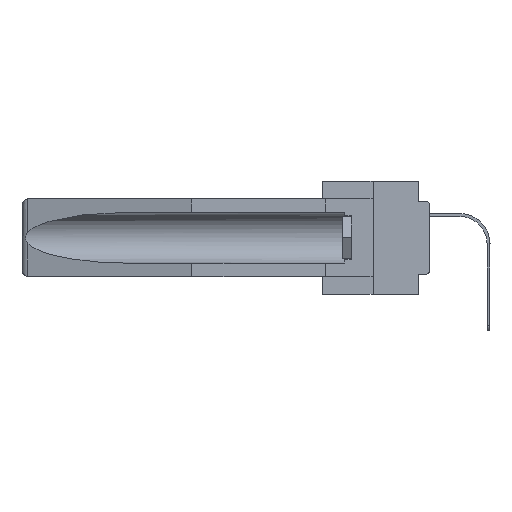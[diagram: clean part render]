
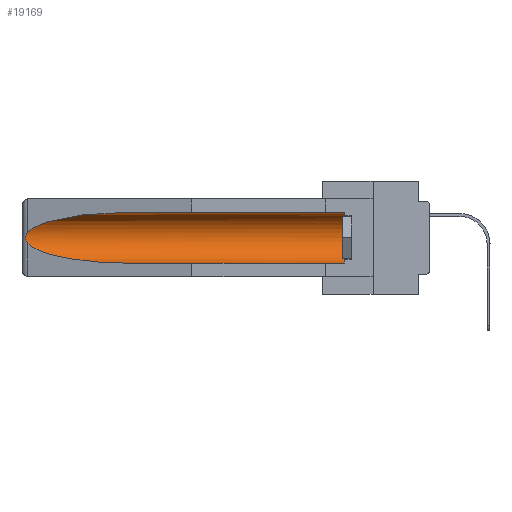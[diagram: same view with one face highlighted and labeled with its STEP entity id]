
A CAD part, left-side view. The second image highlights one B-rep face of the part: STEP entity #19169.
In plain terms, the highlighted cylindrical face has radius 2.857 mm (diameter 5.715 mm), a partial arc.
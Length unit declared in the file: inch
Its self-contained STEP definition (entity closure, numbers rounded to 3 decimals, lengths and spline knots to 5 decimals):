
#173 = CARTESIAN_POINT ( 'NONE',  ( 0.26537, 1.52718, -0.14972 ) ) ;
#733 = CARTESIAN_POINT ( 'NONE',  ( 0.26537, 1.52718, -0.19328 ) ) ;
#929 = ORIENTED_EDGE ( 'NONE', *, *, #22819, .T. ) ;
#1389 = CARTESIAN_POINT ( 'NONE',  ( 0.155, 0.126, -0.059 ) ) ;
#3145 = CARTESIAN_POINT ( 'NONE',  ( 0.155, -0.30754, -0.059 ) ) ;
#3261 = AXIS2_PLACEMENT_3D ( 'NONE', #9724, #14169, #6848 ) ;
#3424 = CARTESIAN_POINT ( 'NONE',  ( 0.25451, 1.48313, -0.24835 ) ) ;
#4746 = ORIENTED_EDGE ( 'NONE', *, *, #31043, .T. ) ;
#5028 = EDGE_CURVE ( 'NONE', #8423, #15513, #22191, .T. ) ;
#6464 = CARTESIAN_POINT ( 'NONE',  ( 0.26537, 1.52718, -0.14972 ) ) ;
#6481 = B_SPLINE_CURVE_WITH_KNOTS ( 'NONE', 3,
 ( #173, #19925, #7110, #12039, #9827, #9662, #19304, #28943, #26724, #24352 ),
 .UNSPECIFIED., .F., .F.,
 ( 4, 2, 2, 2, 4 ),
 ( 0., 0.00029, 0.00058, 0.00087, 0.00117 ),
 .UNSPECIFIED. ) ;
#6804 = CARTESIAN_POINT ( 'NONE',  ( 0.155, 0.126, -0.1715 ) ) ;
#6848 = DIRECTION ( 'NONE',  ( 0., 0., 1. ) ) ;
#7110 = CARTESIAN_POINT ( 'NONE',  ( 0.26654, 1.53092, -0.15636 ) ) ;
#8216 = VECTOR ( 'NONE', #19935, 39.37008 ) ;
#8423 = VERTEX_POINT ( 'NONE', #8810 ) ;
#8810 = CARTESIAN_POINT ( 'NONE',  ( 0.155, 1.07973, -0.059 ) ) ;
#8947 = ORIENTED_EDGE ( 'NONE', *, *, #17064, .T. ) ;
#9302 = CARTESIAN_POINT ( 'NONE',  ( 0.26537, 1.52718, -0.14972 ) ) ;
#9662 = CARTESIAN_POINT ( 'NONE',  ( 0.2675, 1.53308, -0.17534 ) ) ;
#9724 = CARTESIAN_POINT ( 'NONE',  ( 0.155, -0.30754, -0.1715 ) ) ;
#9750 = DIRECTION ( 'NONE',  ( 0., 1., 0. ) ) ;
#9827 = CARTESIAN_POINT ( 'NONE',  ( 0.2675, 1.53308, -0.16763 ) ) ;
#10539 = EDGE_LOOP ( 'NONE', ( #30021, #11380, #8947, #20277, #4746, #929 ) ) ;
#11380 = ORIENTED_EDGE ( 'NONE', *, *, #29984, .T. ) ;
#12039 = CARTESIAN_POINT ( 'NONE',  ( 0.2673, 1.5327, -0.16383 ) ) ;
#12760 = VERTEX_POINT ( 'NONE', #13116 ) ;
#12958 = CARTESIAN_POINT ( 'NONE',  ( 0.26537, 1.52718, -0.19328 ) ) ;
#13102 = CARTESIAN_POINT ( 'NONE',  ( 0.155, 1.07973, -0.284 ) ) ;
#13116 = CARTESIAN_POINT ( 'NONE',  ( 0.155, 0.126, -0.284 ) ) ;
#13557 = CIRCLE ( 'NONE', #17582, 0.1125 ) ;
#14154 = VERTEX_POINT ( 'NONE', #16433 ) ;
#14169 = DIRECTION ( 'NONE',  ( 0., 1., 0. ) ) ;
#15513 = VERTEX_POINT ( 'NONE', #9302 ) ;
#16433 = CARTESIAN_POINT ( 'NONE',  ( 0.155, 1.07973, -0.284 ) ) ;
#16639 = DIRECTION ( 'NONE',  ( 0., -1., 0. ) ) ;
#17064 = EDGE_CURVE ( 'NONE', #25008, #14154, #19153, .T. ) ;
#17582 = AXIS2_PLACEMENT_3D ( 'NONE', #6804, #16639, #26437 ) ;
#19153 =( BOUNDED_CURVE ( )  B_SPLINE_CURVE ( 3, ( #12958, #3424, #27639, #13102 ),
 .UNSPECIFIED., .F., .F. ) 
 B_SPLINE_CURVE_WITH_KNOTS ( ( 4, 4 ),
 ( 0.1948, 1.5708 ),
 .UNSPECIFIED. ) 
 CURVE ( )  GEOMETRIC_REPRESENTATION_ITEM ( )  RATIONAL_B_SPLINE_CURVE ( ( 1., 0.848, 0.848, 1. ) ) 
 REPRESENTATION_ITEM ( '' )  );
#19169 = ADVANCED_FACE ( 'NONE', ( #30881 ), #23627, .F. ) ;
#19304 = CARTESIAN_POINT ( 'NONE',  ( 0.2673, 1.53269, -0.17917 ) ) ;
#19394 = LINE ( 'NONE', #24120, #20798 ) ;
#19925 = CARTESIAN_POINT ( 'NONE',  ( 0.26597, 1.52961, -0.15275 ) ) ;
#19935 = DIRECTION ( 'NONE',  ( 0., 1., 0. ) ) ;
#20277 = ORIENTED_EDGE ( 'NONE', *, *, #22202, .F. ) ;
#20798 = VECTOR ( 'NONE', #9750, 39.37008 ) ;
#20894 = CARTESIAN_POINT ( 'NONE',  ( 0.155, 1.07973, -0.059 ) ) ;
#22191 =( BOUNDED_CURVE ( )  B_SPLINE_CURVE ( 3, ( #20894, #30510, #28158, #6464 ),
 .UNSPECIFIED., .F., .F. ) 
 B_SPLINE_CURVE_WITH_KNOTS ( ( 4, 4 ),
 ( 4.71239, 6.08839 ),
 .UNSPECIFIED. ) 
 CURVE ( )  GEOMETRIC_REPRESENTATION_ITEM ( )  RATIONAL_B_SPLINE_CURVE ( ( 1., 0.848, 0.848, 1. ) ) 
 REPRESENTATION_ITEM ( '' )  );
#22202 = EDGE_CURVE ( 'NONE', #12760, #14154, #19394, .T. ) ;
#22819 = EDGE_CURVE ( 'NONE', #30105, #8423, #24999, .T. ) ;
#23627 = CYLINDRICAL_SURFACE ( 'NONE', #3261, 0.1125 ) ;
#24120 = CARTESIAN_POINT ( 'NONE',  ( 0.155, -0.30754, -0.284 ) ) ;
#24352 = CARTESIAN_POINT ( 'NONE',  ( 0.26537, 1.52718, -0.19328 ) ) ;
#24999 = LINE ( 'NONE', #3145, #8216 ) ;
#25008 = VERTEX_POINT ( 'NONE', #733 ) ;
#26437 = DIRECTION ( 'NONE',  ( 0., 0., 1. ) ) ;
#26724 = CARTESIAN_POINT ( 'NONE',  ( 0.26597, 1.5296, -0.19026 ) ) ;
#27639 = CARTESIAN_POINT ( 'NONE',  ( 0.21114, 1.30732, -0.284 ) ) ;
#28158 = CARTESIAN_POINT ( 'NONE',  ( 0.25451, 1.48313, -0.09465 ) ) ;
#28943 = CARTESIAN_POINT ( 'NONE',  ( 0.26655, 1.53094, -0.18657 ) ) ;
#29984 = EDGE_CURVE ( 'NONE', #15513, #25008, #6481, .T. ) ;
#30021 = ORIENTED_EDGE ( 'NONE', *, *, #5028, .T. ) ;
#30105 = VERTEX_POINT ( 'NONE', #1389 ) ;
#30510 = CARTESIAN_POINT ( 'NONE',  ( 0.21114, 1.30732, -0.059 ) ) ;
#30881 = FACE_OUTER_BOUND ( 'NONE', #10539, .T. ) ;
#31043 = EDGE_CURVE ( 'NONE', #12760, #30105, #13557, .T. ) ;
